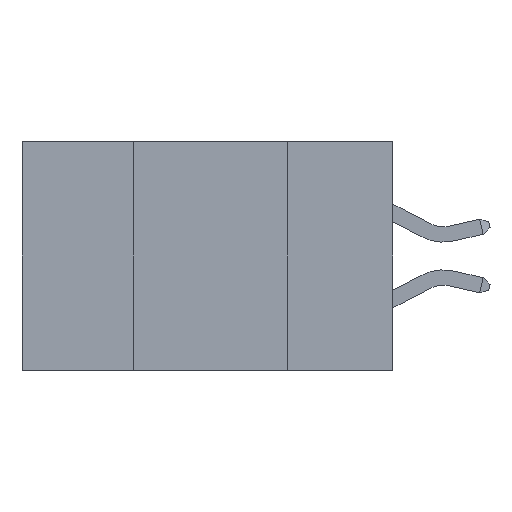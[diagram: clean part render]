
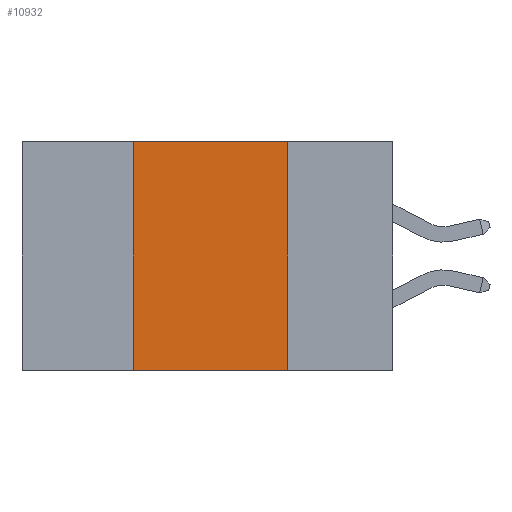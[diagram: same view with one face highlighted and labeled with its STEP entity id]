
A CAD part, left-side view. The second image highlights one B-rep face of the part: STEP entity #10932.
In plain terms, the highlighted planar face has unit normal (-1, 0, 0).
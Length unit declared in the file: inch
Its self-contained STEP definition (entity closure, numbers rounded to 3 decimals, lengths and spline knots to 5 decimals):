
#170 = EDGE_CURVE ( 'NONE', #12313, #15793, #6411, .T. ) ;
#384 = CARTESIAN_POINT ( 'NONE',  ( 0., 0.42, 0. ) ) ;
#409 = ORIENTED_EDGE ( 'NONE', *, *, #17574, .T. ) ;
#1701 = CARTESIAN_POINT ( 'NONE',  ( 0., 0.17, 0. ) ) ;
#2897 = DIRECTION ( 'NONE',  ( 1., 0., 0. ) ) ;
#4274 = LINE ( 'NONE', #11551, #16197 ) ;
#4403 = FACE_OUTER_BOUND ( 'NONE', #18872, .T. ) ;
#5874 = CARTESIAN_POINT ( 'NONE',  ( 0., 0.42, 0. ) ) ;
#6411 = LINE ( 'NONE', #384, #15071 ) ;
#6576 = LINE ( 'NONE', #11139, #14293 ) ;
#7162 = LINE ( 'NONE', #9175, #18798 ) ;
#7740 = DIRECTION ( 'NONE',  ( 0., -1., 0. ) ) ;
#9175 = CARTESIAN_POINT ( 'NONE',  ( 0., 0.6, 0. ) ) ;
#9611 = CARTESIAN_POINT ( 'NONE',  ( 0., 0.6, 0. ) ) ;
#9841 = DIRECTION ( 'NONE',  ( 0., 0., -1. ) ) ;
#9851 = ORIENTED_EDGE ( 'NONE', *, *, #15775, .F. ) ;
#10153 = ORIENTED_EDGE ( 'NONE', *, *, #13540, .F. ) ;
#10190 = ORIENTED_EDGE ( 'NONE', *, *, #170, .F. ) ;
#10932 = ADVANCED_FACE ( 'NONE', ( #4403 ), #12951, .F. ) ;
#11139 = CARTESIAN_POINT ( 'NONE',  ( 0., 0.6, -0.37 ) ) ;
#11551 = CARTESIAN_POINT ( 'NONE',  ( 0., 0.17, 0. ) ) ;
#12313 = VERTEX_POINT ( 'NONE', #16236 ) ;
#12629 = DIRECTION ( 'NONE',  ( 0., -1., 0. ) ) ;
#12951 = PLANE ( 'NONE',  #19538 ) ;
#13540 = EDGE_CURVE ( 'NONE', #17212, #13983, #4274, .T. ) ;
#13983 = VERTEX_POINT ( 'NONE', #20132 ) ;
#14293 = VECTOR ( 'NONE', #7740, 39.37008 ) ;
#14477 = DIRECTION ( 'NONE',  ( 0., 0., -1. ) ) ;
#15071 = VECTOR ( 'NONE', #17102, 39.37008 ) ;
#15775 = EDGE_CURVE ( 'NONE', #15793, #17212, #7162, .T. ) ;
#15793 = VERTEX_POINT ( 'NONE', #5874 ) ;
#16197 = VECTOR ( 'NONE', #9841, 39.37008 ) ;
#16236 = CARTESIAN_POINT ( 'NONE',  ( 0., 0.42, -0.37 ) ) ;
#17102 = DIRECTION ( 'NONE',  ( 0., 0., 1. ) ) ;
#17212 = VERTEX_POINT ( 'NONE', #1701 ) ;
#17574 = EDGE_CURVE ( 'NONE', #12313, #13983, #6576, .T. ) ;
#18798 = VECTOR ( 'NONE', #12629, 39.37008 ) ;
#18872 = EDGE_LOOP ( 'NONE', ( #10153, #9851, #10190, #409 ) ) ;
#19538 = AXIS2_PLACEMENT_3D ( 'NONE', #9611, #2897, #14477 ) ;
#20132 = CARTESIAN_POINT ( 'NONE',  ( 0., 0.17, -0.37 ) ) ;
